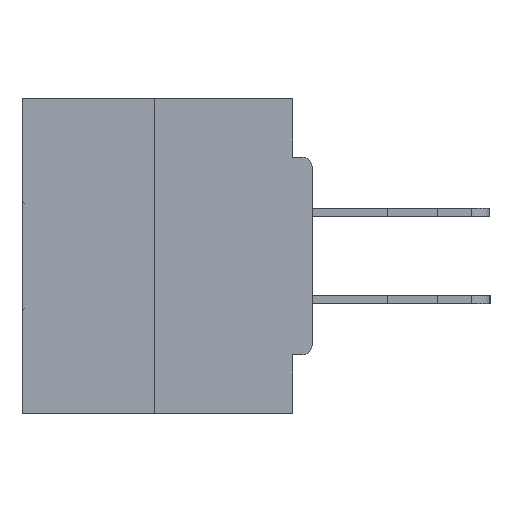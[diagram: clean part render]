
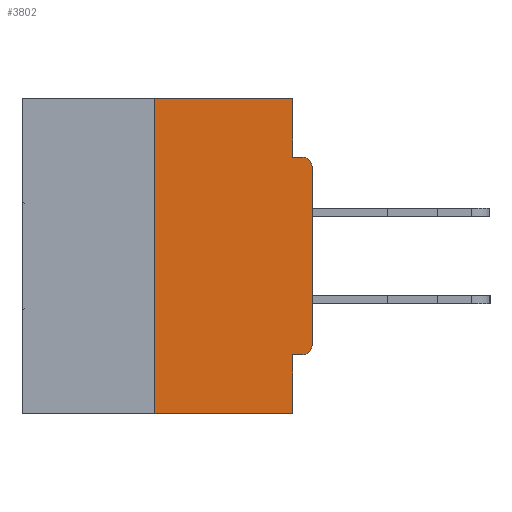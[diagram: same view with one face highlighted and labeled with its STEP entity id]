
A CAD part, left-side view. The second image highlights one B-rep face of the part: STEP entity #3802.
In plain terms, the highlighted planar face has unit normal (-1, 0, 0).
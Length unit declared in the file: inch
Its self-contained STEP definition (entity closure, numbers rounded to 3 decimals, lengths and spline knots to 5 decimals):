
#469 = VERTEX_POINT ( 'NONE', #672 ) ;
#627 = VECTOR ( 'NONE', #26684, 39.37008 ) ;
#672 = CARTESIAN_POINT ( 'NONE',  ( 0., 0.031, -0.5 ) ) ;
#2490 = VERTEX_POINT ( 'NONE', #6241 ) ;
#2974 = EDGE_CURVE ( 'NONE', #27258, #31389, #17923, .T. ) ;
#3680 = CARTESIAN_POINT ( 'NONE',  ( 0., 0., -0.1085 ) ) ;
#3787 = CARTESIAN_POINT ( 'NONE',  ( 0., 0.46, 0. ) ) ;
#3802 = ADVANCED_FACE ( 'NONE', ( #40212 ), #10597, .F. ) ;
#3903 = CARTESIAN_POINT ( 'NONE',  ( 0., 0.46, -0.5 ) ) ;
#4238 = CARTESIAN_POINT ( 'NONE',  ( 0., 0.25, 0. ) ) ;
#4270 = CIRCLE ( 'NONE', #21962, 0.015 ) ;
#4278 = DIRECTION ( 'NONE',  ( -1., 0., 0. ) ) ;
#4664 = LINE ( 'NONE', #4238, #6193 ) ;
#4754 = CARTESIAN_POINT ( 'NONE',  ( 0., 0.031, 0. ) ) ;
#5986 = CARTESIAN_POINT ( 'NONE',  ( 0., 0.015, -0.1085 ) ) ;
#6193 = VECTOR ( 'NONE', #17872, 39.37008 ) ;
#6241 = CARTESIAN_POINT ( 'NONE',  ( 0., 0.25, 0. ) ) ;
#6359 = LINE ( 'NONE', #38966, #21908 ) ;
#7313 = EDGE_CURVE ( 'NONE', #11864, #28987, #14236, .T. ) ;
#9823 = LINE ( 'NONE', #22826, #10970 ) ;
#10509 = ORIENTED_EDGE ( 'NONE', *, *, #34442, .F. ) ;
#10597 = PLANE ( 'NONE',  #40926 ) ;
#10970 = VECTOR ( 'NONE', #36629, 39.37008 ) ;
#11323 = LINE ( 'NONE', #24318, #21334 ) ;
#11541 = LINE ( 'NONE', #34935, #19057 ) ;
#11808 = AXIS2_PLACEMENT_3D ( 'NONE', #5986, #35367, #19392 ) ;
#11864 = VERTEX_POINT ( 'NONE', #36981 ) ;
#12784 = EDGE_CURVE ( 'NONE', #19297, #469, #16677, .T. ) ;
#13506 = EDGE_CURVE ( 'NONE', #22912, #34086, #11541, .T. ) ;
#13516 = ORIENTED_EDGE ( 'NONE', *, *, #26524, .F. ) ;
#14236 = LINE ( 'NONE', #20621, #17523 ) ;
#14450 = DIRECTION ( 'NONE',  ( 0., 1., 0. ) ) ;
#15492 = EDGE_CURVE ( 'NONE', #28987, #469, #6359, .T. ) ;
#16132 = ORIENTED_EDGE ( 'NONE', *, *, #15492, .F. ) ;
#16626 = CARTESIAN_POINT ( 'NONE',  ( 0., 0.031, -0.4065 ) ) ;
#16677 = LINE ( 'NONE', #3903, #627 ) ;
#17523 = VECTOR ( 'NONE', #14450, 39.37008 ) ;
#17709 = DIRECTION ( 'NONE',  ( 0., 0., -1. ) ) ;
#17872 = DIRECTION ( 'NONE',  ( 0., 0., 1. ) ) ;
#17923 = CIRCLE ( 'NONE', #11808, 0.015 ) ;
#18009 = ORIENTED_EDGE ( 'NONE', *, *, #12784, .T. ) ;
#18452 = CARTESIAN_POINT ( 'NONE',  ( 0., 0., -0.0935 ) ) ;
#19057 = VECTOR ( 'NONE', #38156, 39.37008 ) ;
#19297 = VERTEX_POINT ( 'NONE', #22791 ) ;
#19347 = DIRECTION ( 'NONE',  ( 0., 0., -1. ) ) ;
#19392 = DIRECTION ( 'NONE',  ( 0., 0., -1. ) ) ;
#19971 = DIRECTION ( 'NONE',  ( 0., 0., -1. ) ) ;
#20189 = DIRECTION ( 'NONE',  ( 1., 0., 0. ) ) ;
#20621 = CARTESIAN_POINT ( 'NONE',  ( 0., 0., -0.4065 ) ) ;
#21334 = VECTOR ( 'NONE', #37294, 39.37008 ) ;
#21908 = VECTOR ( 'NONE', #19347, 39.37008 ) ;
#21962 = AXIS2_PLACEMENT_3D ( 'NONE', #30891, #4278, #17709 ) ;
#22791 = CARTESIAN_POINT ( 'NONE',  ( 0., 0.25, -0.5 ) ) ;
#22826 = CARTESIAN_POINT ( 'NONE',  ( 0., 0.46, 0. ) ) ;
#22912 = VERTEX_POINT ( 'NONE', #4754 ) ;
#24318 = CARTESIAN_POINT ( 'NONE',  ( 0., 0., 0. ) ) ;
#24355 = CARTESIAN_POINT ( 'NONE',  ( 0., 0.015, -0.0935 ) ) ;
#24425 = ORIENTED_EDGE ( 'NONE', *, *, #37356, .F. ) ;
#25797 = ORIENTED_EDGE ( 'NONE', *, *, #13506, .F. ) ;
#26524 = EDGE_CURVE ( 'NONE', #34086, #31389, #36971, .T. ) ;
#26684 = DIRECTION ( 'NONE',  ( 0., -1., 0. ) ) ;
#27258 = VERTEX_POINT ( 'NONE', #3680 ) ;
#28025 = DIRECTION ( 'NONE',  ( 0., -1., 0. ) ) ;
#28380 = CARTESIAN_POINT ( 'NONE',  ( 0., 0., -0.3915 ) ) ;
#28884 = EDGE_LOOP ( 'NONE', ( #24425, #10509, #18009, #16132, #40118, #34015, #34288, #30273, #13516, #25797 ) ) ;
#28987 = VERTEX_POINT ( 'NONE', #16626 ) ;
#30273 = ORIENTED_EDGE ( 'NONE', *, *, #2974, .T. ) ;
#30891 = CARTESIAN_POINT ( 'NONE',  ( 0., 0.015, -0.3915 ) ) ;
#31389 = VERTEX_POINT ( 'NONE', #24355 ) ;
#31751 = CARTESIAN_POINT ( 'NONE',  ( 0., 0.031, -0.0935 ) ) ;
#34015 = ORIENTED_EDGE ( 'NONE', *, *, #38824, .T. ) ;
#34086 = VERTEX_POINT ( 'NONE', #31751 ) ;
#34288 = ORIENTED_EDGE ( 'NONE', *, *, #41396, .T. ) ;
#34442 = EDGE_CURVE ( 'NONE', #19297, #2490, #4664, .T. ) ;
#34935 = CARTESIAN_POINT ( 'NONE',  ( 0., 0.031, 0. ) ) ;
#35367 = DIRECTION ( 'NONE',  ( -1., 0., 0. ) ) ;
#36369 = VECTOR ( 'NONE', #28025, 39.37008 ) ;
#36629 = DIRECTION ( 'NONE',  ( 0., -1., 0. ) ) ;
#36971 = LINE ( 'NONE', #18452, #36369 ) ;
#36981 = CARTESIAN_POINT ( 'NONE',  ( 0., 0.015, -0.4065 ) ) ;
#37294 = DIRECTION ( 'NONE',  ( 0., 0., 1. ) ) ;
#37356 = EDGE_CURVE ( 'NONE', #2490, #22912, #9823, .T. ) ;
#38156 = DIRECTION ( 'NONE',  ( 0., 0., -1. ) ) ;
#38551 = VERTEX_POINT ( 'NONE', #28380 ) ;
#38824 = EDGE_CURVE ( 'NONE', #11864, #38551, #4270, .T. ) ;
#38966 = CARTESIAN_POINT ( 'NONE',  ( 0., 0.031, -0.5 ) ) ;
#40118 = ORIENTED_EDGE ( 'NONE', *, *, #7313, .F. ) ;
#40212 = FACE_OUTER_BOUND ( 'NONE', #28884, .T. ) ;
#40926 = AXIS2_PLACEMENT_3D ( 'NONE', #3787, #20189, #19971 ) ;
#41396 = EDGE_CURVE ( 'NONE', #38551, #27258, #11323, .T. ) ;
